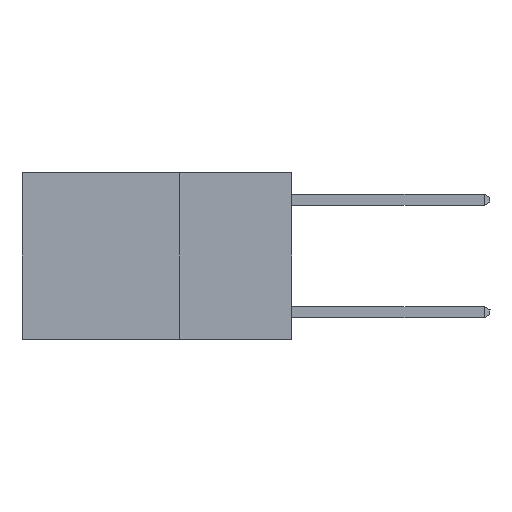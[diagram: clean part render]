
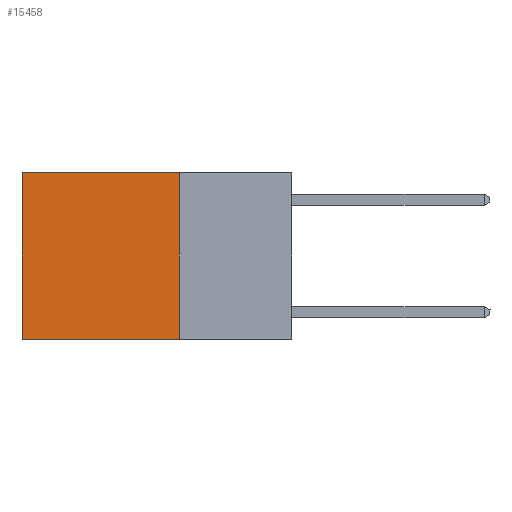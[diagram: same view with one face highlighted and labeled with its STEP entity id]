
A CAD part, left-side view. The second image highlights one B-rep face of the part: STEP entity #15458.
In plain terms, the highlighted planar face has unit normal (-1, 0, 0).
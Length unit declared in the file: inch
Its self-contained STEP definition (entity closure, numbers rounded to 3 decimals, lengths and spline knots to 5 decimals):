
#1011 = VECTOR ( 'NONE', #6904, 39.37008 ) ;
#1239 = VERTEX_POINT ( 'NONE', #16317 ) ;
#1377 = CARTESIAN_POINT ( 'NONE',  ( 0.2625, 0.25, 0. ) ) ;
#1572 = VECTOR ( 'NONE', #6127, 39.37008 ) ;
#3100 = CARTESIAN_POINT ( 'NONE',  ( 0.2625, 0.6, 0. ) ) ;
#3390 = EDGE_CURVE ( 'NONE', #1239, #4113, #4659, .T. ) ;
#3599 = VERTEX_POINT ( 'NONE', #11305 ) ;
#3692 = CARTESIAN_POINT ( 'NONE',  ( 0.2625, 0.25, 0. ) ) ;
#4113 = VERTEX_POINT ( 'NONE', #18391 ) ;
#4526 = CARTESIAN_POINT ( 'NONE',  ( 0.2625, 0.6, 0. ) ) ;
#4659 = LINE ( 'NONE', #1377, #12524 ) ;
#5675 = EDGE_LOOP ( 'NONE', ( #16708, #17051, #17093, #17285 ) ) ;
#5873 = DIRECTION ( 'NONE',  ( 0., 0., -1. ) ) ;
#6127 = DIRECTION ( 'NONE',  ( 0., 0., -1. ) ) ;
#6737 = EDGE_CURVE ( 'NONE', #1239, #10054, #9515, .T. ) ;
#6904 = DIRECTION ( 'NONE',  ( 0., 1., 0. ) ) ;
#9515 = LINE ( 'NONE', #3692, #1011 ) ;
#10054 = VERTEX_POINT ( 'NONE', #3100 ) ;
#10404 = EDGE_CURVE ( 'NONE', #4113, #3599, #16196, .T. ) ;
#10538 = LINE ( 'NONE', #4526, #1572 ) ;
#11305 = CARTESIAN_POINT ( 'NONE',  ( 0.2625, 0.6, -0.37 ) ) ;
#11884 = DIRECTION ( 'NONE',  ( 0., 1., 0. ) ) ;
#11899 = AXIS2_PLACEMENT_3D ( 'NONE', #12124, #15069, #5873 ) ;
#12124 = CARTESIAN_POINT ( 'NONE',  ( 0.2625, 0.25, 0. ) ) ;
#12524 = VECTOR ( 'NONE', #18237, 39.37008 ) ;
#13506 = FACE_OUTER_BOUND ( 'NONE', #5675, .T. ) ;
#15069 = DIRECTION ( 'NONE',  ( 1., 0., 0. ) ) ;
#15458 = ADVANCED_FACE ( 'NONE', ( #13506 ), #19236, .F. ) ;
#16196 = LINE ( 'NONE', #19020, #16651 ) ;
#16317 = CARTESIAN_POINT ( 'NONE',  ( 0.2625, 0.25, 0. ) ) ;
#16651 = VECTOR ( 'NONE', #11884, 39.37008 ) ;
#16708 = ORIENTED_EDGE ( 'NONE', *, *, #18794, .T. ) ;
#17051 = ORIENTED_EDGE ( 'NONE', *, *, #10404, .F. ) ;
#17093 = ORIENTED_EDGE ( 'NONE', *, *, #3390, .F. ) ;
#17285 = ORIENTED_EDGE ( 'NONE', *, *, #6737, .T. ) ;
#18237 = DIRECTION ( 'NONE',  ( 0., 0., -1. ) ) ;
#18391 = CARTESIAN_POINT ( 'NONE',  ( 0.2625, 0.25, -0.37 ) ) ;
#18794 = EDGE_CURVE ( 'NONE', #10054, #3599, #10538, .T. ) ;
#19020 = CARTESIAN_POINT ( 'NONE',  ( 0.2625, 0.25, -0.37 ) ) ;
#19236 = PLANE ( 'NONE',  #11899 ) ;
